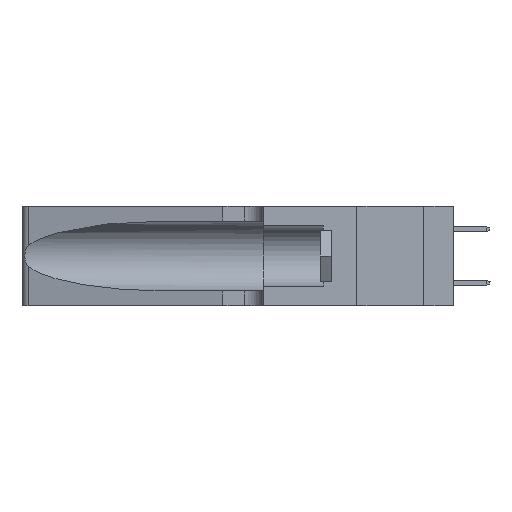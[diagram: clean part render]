
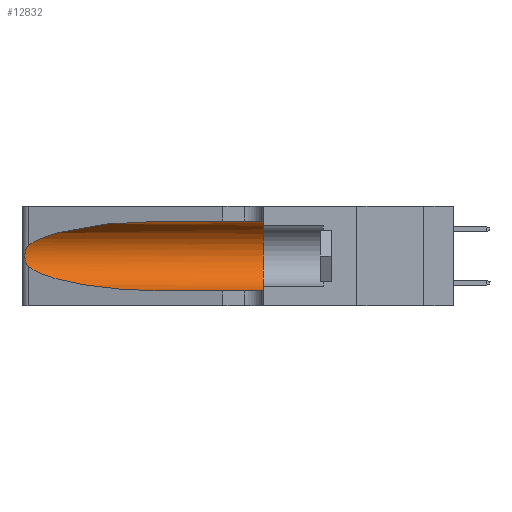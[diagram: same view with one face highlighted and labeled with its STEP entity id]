
A CAD part, left-side view. The second image highlights one B-rep face of the part: STEP entity #12832.
In plain terms, the highlighted cylindrical face has radius 3.308 mm (diameter 6.617 mm), a partial arc.
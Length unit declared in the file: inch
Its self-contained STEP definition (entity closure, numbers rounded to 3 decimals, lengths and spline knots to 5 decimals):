
#71 = ORIENTED_EDGE ( 'NONE', *, *, #17108, .T. ) ;
#352 = VERTEX_POINT ( 'NONE', #6323 ) ;
#626 = EDGE_CURVE ( 'NONE', #12729, #352, #12598, .T. ) ;
#738 = AXIS2_PLACEMENT_3D ( 'NONE', #20095, #2210, #5139 ) ;
#1779 = EDGE_LOOP ( 'NONE', ( #21433, #9257, #25140, #71, #9689, #20679 ) ) ;
#1890 =( BOUNDED_CURVE ( )  B_SPLINE_CURVE ( 3, ( #31634, #32127, #4094, #11728 ),
 .UNSPECIFIED., .F., .T. ) 
 B_SPLINE_CURVE_WITH_KNOTS ( ( 4, 4 ),
 ( 1.5708, 2.84003 ),
 .UNSPECIFIED. ) 
 CURVE ( )  GEOMETRIC_REPRESENTATION_ITEM ( )  RATIONAL_B_SPLINE_CURVE ( ( 1., 0.87, 0.87, 1. ) ) 
 REPRESENTATION_ITEM ( '' )  );
#2210 = DIRECTION ( 'NONE',  ( 0., 1., 0. ) ) ;
#2586 = CARTESIAN_POINT ( 'NONE',  ( 0.1305, 0.35, 0.05475 ) ) ;
#2702 = EDGE_CURVE ( 'NONE', #18134, #12729, #29947, .T. ) ;
#2846 = CARTESIAN_POINT ( 'NONE',  ( 0.26075, 1.23896, 0.178 ) ) ;
#2900 = FACE_OUTER_BOUND ( 'NONE', #1779, .T. ) ;
#4094 = CARTESIAN_POINT ( 'NONE',  ( 0.2373, 1.15595, 0.28018 ) ) ;
#4939 = CARTESIAN_POINT ( 'NONE',  ( 0.1305, 1.61858, 0.05475 ) ) ;
#5007 = CARTESIAN_POINT ( 'NONE',  ( 0.25487, 1.22718, 0.14631 ) ) ;
#5103 = CARTESIAN_POINT ( 'NONE',  ( 0.25789, 1.23486, 0.15765 ) ) ;
#5139 = DIRECTION ( 'NONE',  ( 0., 0., 1. ) ) ;
#5242 = DIRECTION ( 'NONE',  ( 0., -1., 0. ) ) ;
#6323 = CARTESIAN_POINT ( 'NONE',  ( 0.1305, 0.72297, 0.05475 ) ) ;
#6866 = VECTOR ( 'NONE', #5242, 39.37008 ) ;
#7068 = CARTESIAN_POINT ( 'NONE',  ( 0.1305, 0.72297, 0.05475 ) ) ;
#7237 = CARTESIAN_POINT ( 'NONE',  ( 0.25555, 1.22993, 0.14849 ) ) ;
#7706 = VECTOR ( 'NONE', #12609, 39.37008 ) ;
#7776 = CARTESIAN_POINT ( 'NONE',  ( 0.25854, 1.2359, 0.20912 ) ) ;
#8333 = CYLINDRICAL_SURFACE ( 'NONE', #29552, 0.13025 ) ;
#9257 = ORIENTED_EDGE ( 'NONE', *, *, #2702, .T. ) ;
#9689 = ORIENTED_EDGE ( 'NONE', *, *, #20767, .F. ) ;
#10823 = DIRECTION ( 'NONE',  ( 0., 0., -1. ) ) ;
#11728 = CARTESIAN_POINT ( 'NONE',  ( 0.25487, 1.22718, 0.22369 ) ) ;
#11751 = CARTESIAN_POINT ( 'NONE',  ( 0.25487, 1.22718, 0.14631 ) ) ;
#11986 = VERTEX_POINT ( 'NONE', #31372 ) ;
#12133 = CARTESIAN_POINT ( 'NONE',  ( 0.1305, 0.35, 0.31525 ) ) ;
#12598 =( BOUNDED_CURVE ( )  B_SPLINE_CURVE ( 3, ( #11751, #17357, #32626, #7068 ),
 .UNSPECIFIED., .F., .T. ) 
 B_SPLINE_CURVE_WITH_KNOTS ( ( 4, 4 ),
 ( 3.44316, 4.71239 ),
 .UNSPECIFIED. ) 
 CURVE ( )  GEOMETRIC_REPRESENTATION_ITEM ( )  RATIONAL_B_SPLINE_CURVE ( ( 1., 0.87, 0.87, 1. ) ) 
 REPRESENTATION_ITEM ( '' )  );
#12609 = DIRECTION ( 'NONE',  ( 0., -1., 0. ) ) ;
#12729 = VERTEX_POINT ( 'NONE', #19173 ) ;
#12790 = CARTESIAN_POINT ( 'NONE',  ( 0.25639, 1.23184, 0.21858 ) ) ;
#12832 = ADVANCED_FACE ( 'NONE', ( #2900 ), #8333, .F. ) ;
#12949 = CARTESIAN_POINT ( 'NONE',  ( 0.26017, 1.23833, 0.17102 ) ) ;
#12991 = CARTESIAN_POINT ( 'NONE',  ( 0.1305, 1.61858, 0.185 ) ) ;
#14316 = LINE ( 'NONE', #27712, #7706 ) ;
#15265 = CARTESIAN_POINT ( 'NONE',  ( 0.25487, 1.22718, 0.22369 ) ) ;
#15424 = CARTESIAN_POINT ( 'NONE',  ( 0.26075, 1.23896, 0.19203 ) ) ;
#17108 = EDGE_CURVE ( 'NONE', #352, #24411, #27651, .T. ) ;
#17357 = CARTESIAN_POINT ( 'NONE',  ( 0.2373, 1.15595, 0.08982 ) ) ;
#17906 = CARTESIAN_POINT ( 'NONE',  ( 0.26018, 1.23835, 0.19895 ) ) ;
#18134 = VERTEX_POINT ( 'NONE', #25658 ) ;
#19173 = CARTESIAN_POINT ( 'NONE',  ( 0.25487, 1.22718, 0.14631 ) ) ;
#20095 = CARTESIAN_POINT ( 'NONE',  ( 0.1305, 0.35, 0.185 ) ) ;
#20269 = CARTESIAN_POINT ( 'NONE',  ( 0.25555, 1.22994, 0.2215 ) ) ;
#20679 = ORIENTED_EDGE ( 'NONE', *, *, #26177, .F. ) ;
#20767 = EDGE_CURVE ( 'NONE', #31127, #24411, #30405, .T. ) ;
#21433 = ORIENTED_EDGE ( 'NONE', *, *, #27492, .T. ) ;
#22541 = CARTESIAN_POINT ( 'NONE',  ( 0.25639, 1.23186, 0.15144 ) ) ;
#22696 = CARTESIAN_POINT ( 'NONE',  ( 0.25856, 1.23593, 0.16098 ) ) ;
#23129 = DIRECTION ( 'NONE',  ( 0., -1., 0. ) ) ;
#24411 = VERTEX_POINT ( 'NONE', #2586 ) ;
#25140 = ORIENTED_EDGE ( 'NONE', *, *, #626, .T. ) ;
#25658 = CARTESIAN_POINT ( 'NONE',  ( 0.25487, 1.22718, 0.22369 ) ) ;
#26177 = EDGE_CURVE ( 'NONE', #11986, #31127, #14316, .T. ) ;
#27492 = EDGE_CURVE ( 'NONE', #11986, #18134, #1890, .T. ) ;
#27651 = LINE ( 'NONE', #4939, #6866 ) ;
#27712 = CARTESIAN_POINT ( 'NONE',  ( 0.1305, 1.61858, 0.31525 ) ) ;
#29552 = AXIS2_PLACEMENT_3D ( 'NONE', #12991, #23129, #10823 ) ;
#29947 = B_SPLINE_CURVE_WITH_KNOTS ( 'NONE', 3,
 ( #15265, #20269, #12790, #30544, #7776, #17906, #15424, #2846, #12949, #22696, #5103, #22541, #7237, #5007 ),
 .UNSPECIFIED., .F., .F.,
 ( 4, 2, 2, 2, 2, 2, 4 ),
 ( 0., 0.00027, 0.00053, 0.00107, 0.0016, 0.00187, 0.00214 ),
 .UNSPECIFIED. ) ;
#30405 = CIRCLE ( 'NONE', #738, 0.13025 ) ;
#30544 = CARTESIAN_POINT ( 'NONE',  ( 0.25787, 1.23484, 0.2124 ) ) ;
#31127 = VERTEX_POINT ( 'NONE', #12133 ) ;
#31372 = CARTESIAN_POINT ( 'NONE',  ( 0.1305, 0.72297, 0.31525 ) ) ;
#31634 = CARTESIAN_POINT ( 'NONE',  ( 0.1305, 0.72297, 0.31525 ) ) ;
#32127 = CARTESIAN_POINT ( 'NONE',  ( 0.18966, 0.96281, 0.31525 ) ) ;
#32626 = CARTESIAN_POINT ( 'NONE',  ( 0.18966, 0.96281, 0.05475 ) ) ;
